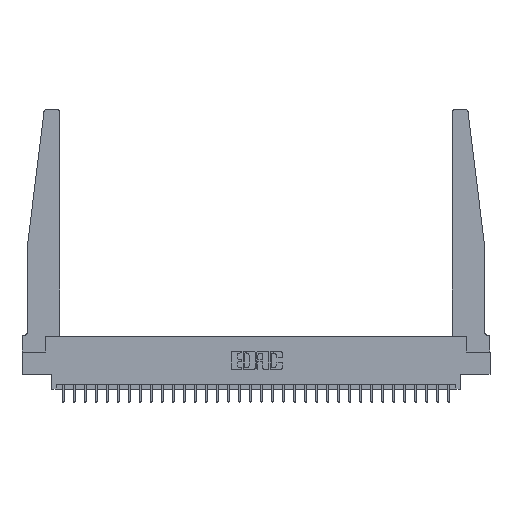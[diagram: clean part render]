
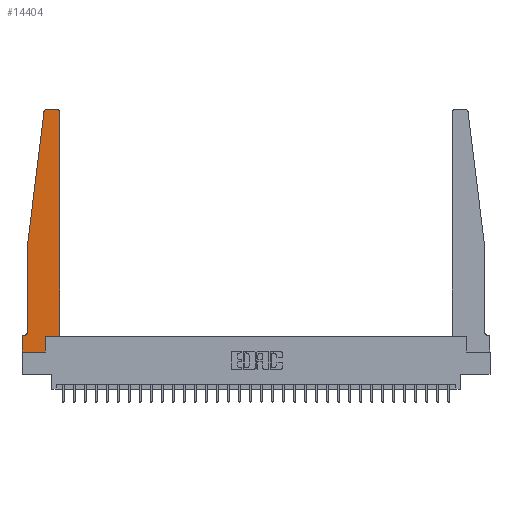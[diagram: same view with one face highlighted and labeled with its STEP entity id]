
A CAD part, top view. The second image highlights one B-rep face of the part: STEP entity #14404.
In plain terms, the highlighted planar face has unit normal (0, 0, 1).
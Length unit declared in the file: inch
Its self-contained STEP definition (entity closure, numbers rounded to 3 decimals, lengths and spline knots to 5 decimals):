
#83 = CARTESIAN_POINT ( 'NONE',  ( 0.395, 2.75, 0.37 ) ) ;
#229 = CARTESIAN_POINT ( 'NONE',  ( 0.065, 0.2375, 0.37 ) ) ;
#282 = ORIENTED_EDGE ( 'NONE', *, *, #18954, .T. ) ;
#636 = EDGE_CURVE ( 'NONE', #9847, #5124, #12114, .T. ) ;
#691 = EDGE_LOOP ( 'NONE', ( #282, #10980, #705, #1917, #1859, #1355, #1486, #882, #977, #9167, #9114, #18964 ) ) ;
#705 = ORIENTED_EDGE ( 'NONE', *, *, #15671, .T. ) ;
#882 = ORIENTED_EDGE ( 'NONE', *, *, #636, .T. ) ;
#977 = ORIENTED_EDGE ( 'NONE', *, *, #8464, .T. ) ;
#1155 = CARTESIAN_POINT ( 'NONE',  ( 0.425, 0.18, 0.37 ) ) ;
#1335 = CARTESIAN_POINT ( 'NONE',  ( 0., 0., 0.37 ) ) ;
#1355 = ORIENTED_EDGE ( 'NONE', *, *, #14274, .T. ) ;
#1486 = ORIENTED_EDGE ( 'NONE', *, *, #3467, .T. ) ;
#1859 = ORIENTED_EDGE ( 'NONE', *, *, #2393, .T. ) ;
#1917 = ORIENTED_EDGE ( 'NONE', *, *, #19083, .T. ) ;
#2188 = DIRECTION ( 'NONE',  ( 0., 0., -1. ) ) ;
#2393 = EDGE_CURVE ( 'NONE', #13939, #18693, #21418, .T. ) ;
#3467 = EDGE_CURVE ( 'NONE', #5454, #9847, #25155, .T. ) ;
#4346 = DIRECTION ( 'NONE',  ( 0., 0., 1. ) ) ;
#4590 = CARTESIAN_POINT ( 'NONE',  ( 0.27653, 2.72, 0.37 ) ) ;
#4827 = EDGE_CURVE ( 'NONE', #22128, #20685, #12147, .T. ) ;
#4934 = CARTESIAN_POINT ( 'NONE',  ( 0., 0., 0.37 ) ) ;
#4999 = VECTOR ( 'NONE', #18812, 39.37008 ) ;
#5124 = VERTEX_POINT ( 'NONE', #11264 ) ;
#5454 = VERTEX_POINT ( 'NONE', #25734 ) ;
#5615 = VECTOR ( 'NONE', #21799, 39.37008 ) ;
#5667 = CARTESIAN_POINT ( 'NONE',  ( 0.065, 1.25, 0.37 ) ) ;
#5775 = DIRECTION ( 'NONE',  ( 1., 0., 0. ) ) ;
#6531 = CARTESIAN_POINT ( 'NONE',  ( 0.27653, 2.75, 0.37 ) ) ;
#6697 = AXIS2_PLACEMENT_3D ( 'NONE', #17990, #4346, #20231 ) ;
#6879 = DIRECTION ( 'NONE',  ( 1., 0., 0. ) ) ;
#7367 = CARTESIAN_POINT ( 'NONE',  ( 0.065, 1.25, 0.37 ) ) ;
#7520 = CARTESIAN_POINT ( 'NONE',  ( 0.425, 2.72, 0.37 ) ) ;
#7552 = VERTEX_POINT ( 'NONE', #7520 ) ;
#7876 = CIRCLE ( 'NONE', #6697, 0.03 ) ;
#8464 = EDGE_CURVE ( 'NONE', #5124, #22128, #13134, .T. ) ;
#8731 = DIRECTION ( 'NONE',  ( 1., 0., 0. ) ) ;
#9114 = ORIENTED_EDGE ( 'NONE', *, *, #13308, .T. ) ;
#9167 = ORIENTED_EDGE ( 'NONE', *, *, #4827, .T. ) ;
#9766 = CARTESIAN_POINT ( 'NONE',  ( 0., 0., 0.37 ) ) ;
#9847 = VERTEX_POINT ( 'NONE', #4934 ) ;
#10466 = VERTEX_POINT ( 'NONE', #83 ) ;
#10980 = ORIENTED_EDGE ( 'NONE', *, *, #13143, .T. ) ;
#11264 = CARTESIAN_POINT ( 'NONE',  ( 0.2605, 0., 0.37 ) ) ;
#11397 = VECTOR ( 'NONE', #8731, 39.37008 ) ;
#11414 = DIRECTION ( 'NONE',  ( 0., 0., 1. ) ) ;
#11433 = VECTOR ( 'NONE', #5775, 39.37008 ) ;
#11809 = AXIS2_PLACEMENT_3D ( 'NONE', #4590, #20469, #6879 ) ;
#12114 = LINE ( 'NONE', #9766, #11397 ) ;
#12147 = LINE ( 'NONE', #1155, #11433 ) ;
#12264 = VERTEX_POINT ( 'NONE', #6531 ) ;
#13134 = LINE ( 'NONE', #17329, #5615 ) ;
#13143 = EDGE_CURVE ( 'NONE', #12264, #20376, #27238, .T. ) ;
#13308 = EDGE_CURVE ( 'NONE', #20685, #7552, #28967, .T. ) ;
#13939 = VERTEX_POINT ( 'NONE', #229 ) ;
#14274 = EDGE_CURVE ( 'NONE', #18693, #5454, #17783, .T. ) ;
#14404 = ADVANCED_FACE ( 'NONE', ( #20219 ), #18154, .T. ) ;
#15256 = CARTESIAN_POINT ( 'NONE',  ( 0.2605, 0.18, 0.37 ) ) ;
#15274 = CARTESIAN_POINT ( 'NONE',  ( 0.24675, 2.72367, 0.37 ) ) ;
#15671 = EDGE_CURVE ( 'NONE', #20376, #20630, #25152, .T. ) ;
#15862 = CARTESIAN_POINT ( 'NONE',  ( 0.015, 0.2375, 0.37 ) ) ;
#16142 = EDGE_CURVE ( 'NONE', #7552, #10466, #7876, .T. ) ;
#16502 = CARTESIAN_POINT ( 'NONE',  ( 0.25, 2.75, 0.37 ) ) ;
#17286 = DIRECTION ( 'NONE',  ( 0., -1., 0. ) ) ;
#17329 = CARTESIAN_POINT ( 'NONE',  ( 0.2605, 0.18, 0.37 ) ) ;
#17783 = LINE ( 'NONE', #21932, #28919 ) ;
#17990 = CARTESIAN_POINT ( 'NONE',  ( 0.395, 2.72, 0.37 ) ) ;
#18135 = DIRECTION ( 'NONE',  ( -1., 0., 0. ) ) ;
#18154 = PLANE ( 'NONE',  #28145 ) ;
#18212 = CARTESIAN_POINT ( 'NONE',  ( 0.065, 1.25, 0.37 ) ) ;
#18406 = CARTESIAN_POINT ( 'NONE',  ( 0.425, 0.18, 0.37 ) ) ;
#18693 = VERTEX_POINT ( 'NONE', #22379 ) ;
#18705 = DIRECTION ( 'NONE',  ( -0.122, -0.992, 0. ) ) ;
#18812 = DIRECTION ( 'NONE',  ( 0., 1., 0. ) ) ;
#18954 = EDGE_CURVE ( 'NONE', #10466, #12264, #21568, .T. ) ;
#18964 = ORIENTED_EDGE ( 'NONE', *, *, #16142, .T. ) ;
#19083 = EDGE_CURVE ( 'NONE', #20630, #13939, #19488, .T. ) ;
#19272 = DIRECTION ( 'NONE',  ( 0., -1., 0. ) ) ;
#19287 = VECTOR ( 'NONE', #17286, 39.37008 ) ;
#19488 = LINE ( 'NONE', #5667, #24672 ) ;
#20219 = FACE_OUTER_BOUND ( 'NONE', #691, .T. ) ;
#20231 = DIRECTION ( 'NONE',  ( 1., 0., 0. ) ) ;
#20376 = VERTEX_POINT ( 'NONE', #15274 ) ;
#20469 = DIRECTION ( 'NONE',  ( 0., 0., 1. ) ) ;
#20630 = VERTEX_POINT ( 'NONE', #18212 ) ;
#20685 = VERTEX_POINT ( 'NONE', #18406 ) ;
#21418 = CIRCLE ( 'NONE', #22164, 0.05 ) ;
#21568 = LINE ( 'NONE', #16502, #27494 ) ;
#21799 = DIRECTION ( 'NONE',  ( 0., 1., 0. ) ) ;
#21932 = CARTESIAN_POINT ( 'NONE',  ( 0.065, 0.1875, 0.37 ) ) ;
#22128 = VERTEX_POINT ( 'NONE', #15256 ) ;
#22164 = AXIS2_PLACEMENT_3D ( 'NONE', #15862, #2188, #18135 ) ;
#22379 = CARTESIAN_POINT ( 'NONE',  ( 0.015, 0.1875, 0.37 ) ) ;
#23241 = CARTESIAN_POINT ( 'NONE',  ( 0.425, 0.18, 0.37 ) ) ;
#24148 = DIRECTION ( 'NONE',  ( -1., 0., 0. ) ) ;
#24455 = VECTOR ( 'NONE', #18705, 39.37008 ) ;
#24672 = VECTOR ( 'NONE', #19272, 39.37008 ) ;
#24824 = CARTESIAN_POINT ( 'NONE',  ( 0., 0.1875, 0.37 ) ) ;
#25152 = LINE ( 'NONE', #7367, #24455 ) ;
#25155 = LINE ( 'NONE', #1335, #19287 ) ;
#25370 = DIRECTION ( 'NONE',  ( -1., 0., 0. ) ) ;
#25734 = CARTESIAN_POINT ( 'NONE',  ( 0., 0.1875, 0.37 ) ) ;
#27098 = DIRECTION ( 'NONE',  ( 1., 0., 0. ) ) ;
#27238 = CIRCLE ( 'NONE', #11809, 0.03 ) ;
#27494 = VECTOR ( 'NONE', #25370, 39.37008 ) ;
#28145 = AXIS2_PLACEMENT_3D ( 'NONE', #24824, #11414, #27098 ) ;
#28919 = VECTOR ( 'NONE', #24148, 39.37008 ) ;
#28967 = LINE ( 'NONE', #23241, #4999 ) ;
